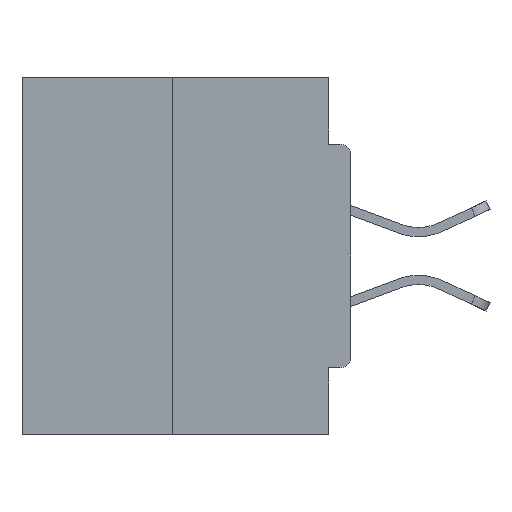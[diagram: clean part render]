
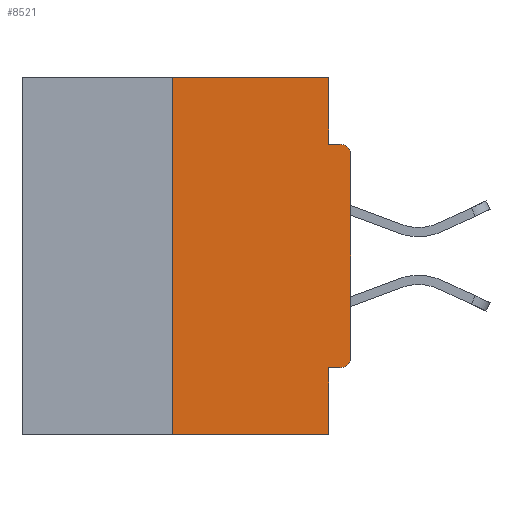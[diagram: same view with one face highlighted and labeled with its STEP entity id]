
A CAD part, left-side view. The second image highlights one B-rep face of the part: STEP entity #8521.
In plain terms, the highlighted planar face has unit normal (-1, 0, 0).
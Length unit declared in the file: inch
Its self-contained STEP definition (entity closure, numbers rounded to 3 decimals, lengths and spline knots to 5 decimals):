
#518 = LINE ( 'NONE', #33857, #13847 ) ;
#1133 = LINE ( 'NONE', #15920, #9068 ) ;
#1143 = CARTESIAN_POINT ( 'NONE',  ( 0., 0.031, -0.0935 ) ) ;
#1361 = VERTEX_POINT ( 'NONE', #1143 ) ;
#1629 = VECTOR ( 'NONE', #17990, 39.37008 ) ;
#2027 = EDGE_CURVE ( 'NONE', #19918, #19166, #31286, .T. ) ;
#2174 = CARTESIAN_POINT ( 'NONE',  ( 0., 0.015, -0.4065 ) ) ;
#2685 = DIRECTION ( 'NONE',  ( 0., 0., 1. ) ) ;
#2753 = DIRECTION ( 'NONE',  ( 0., 1., 0. ) ) ;
#2763 = FACE_OUTER_BOUND ( 'NONE', #19961, .T. ) ;
#3232 = ORIENTED_EDGE ( 'NONE', *, *, #8965, .T. ) ;
#3817 = ORIENTED_EDGE ( 'NONE', *, *, #30612, .F. ) ;
#4650 = CARTESIAN_POINT ( 'NONE',  ( 0., 0.25, -0.5 ) ) ;
#4652 = ORIENTED_EDGE ( 'NONE', *, *, #2027, .T. ) ;
#4657 = CARTESIAN_POINT ( 'NONE',  ( 0., 0.031, 0. ) ) ;
#4737 = DIRECTION ( 'NONE',  ( 0., -1., 0. ) ) ;
#4924 = EDGE_CURVE ( 'NONE', #19918, #27239, #34096, .T. ) ;
#4935 = CARTESIAN_POINT ( 'NONE',  ( 0., 0.031, -0.5 ) ) ;
#5098 = VERTEX_POINT ( 'NONE', #27482 ) ;
#7703 = EDGE_CURVE ( 'NONE', #1361, #5098, #30983, .T. ) ;
#7710 = CARTESIAN_POINT ( 'NONE',  ( 0., 0.46, 0. ) ) ;
#7733 = DIRECTION ( 'NONE',  ( 0., 0., -1. ) ) ;
#8521 = ADVANCED_FACE ( 'NONE', ( #2763 ), #30491, .F. ) ;
#8965 = EDGE_CURVE ( 'NONE', #17860, #16207, #21407, .T. ) ;
#9068 = VECTOR ( 'NONE', #2685, 39.37008 ) ;
#9953 = ORIENTED_EDGE ( 'NONE', *, *, #4924, .F. ) ;
#10108 = DIRECTION ( 'NONE',  ( 0., -1., 0. ) ) ;
#10559 = VECTOR ( 'NONE', #4737, 39.37008 ) ;
#11666 = CARTESIAN_POINT ( 'NONE',  ( 0., 0.031, -0.5 ) ) ;
#12344 = VECTOR ( 'NONE', #16666, 39.37008 ) ;
#12427 = EDGE_CURVE ( 'NONE', #32686, #5098, #20675, .T. ) ;
#13296 = DIRECTION ( 'NONE',  ( 0., 0., -1. ) ) ;
#13358 = CARTESIAN_POINT ( 'NONE',  ( 0., 0.031, -0.4065 ) ) ;
#13772 = ORIENTED_EDGE ( 'NONE', *, *, #26537, .T. ) ;
#13847 = VECTOR ( 'NONE', #10108, 39.37008 ) ;
#14230 = CARTESIAN_POINT ( 'NONE',  ( 0., 0., -0.0935 ) ) ;
#15646 = CARTESIAN_POINT ( 'NONE',  ( 0., 0., -0.4065 ) ) ;
#15920 = CARTESIAN_POINT ( 'NONE',  ( 0., 0., 0. ) ) ;
#16140 = ORIENTED_EDGE ( 'NONE', *, *, #32725, .F. ) ;
#16207 = VERTEX_POINT ( 'NONE', #24730 ) ;
#16448 = AXIS2_PLACEMENT_3D ( 'NONE', #7710, #28440, #20427 ) ;
#16666 = DIRECTION ( 'NONE',  ( 0., -1., 0. ) ) ;
#17650 = VECTOR ( 'NONE', #7733, 39.37008 ) ;
#17860 = VERTEX_POINT ( 'NONE', #2174 ) ;
#17990 = DIRECTION ( 'NONE',  ( 0., 0., -1. ) ) ;
#18476 = ORIENTED_EDGE ( 'NONE', *, *, #28109, .F. ) ;
#19166 = VERTEX_POINT ( 'NONE', #11666 ) ;
#19566 = ORIENTED_EDGE ( 'NONE', *, *, #12427, .T. ) ;
#19918 = VERTEX_POINT ( 'NONE', #4650 ) ;
#19961 = EDGE_LOOP ( 'NONE', ( #23922, #9953, #4652, #18476, #16140, #3232, #13772, #19566, #20881, #3817 ) ) ;
#20427 = DIRECTION ( 'NONE',  ( 0., 0., -1. ) ) ;
#20675 = CIRCLE ( 'NONE', #26813, 0.015 ) ;
#20879 = DIRECTION ( 'NONE',  ( 0., 0., 1. ) ) ;
#20881 = ORIENTED_EDGE ( 'NONE', *, *, #7703, .F. ) ;
#21407 = CIRCLE ( 'NONE', #23380, 0.015 ) ;
#22121 = CARTESIAN_POINT ( 'NONE',  ( 0., 0.031, 0. ) ) ;
#23380 = AXIS2_PLACEMENT_3D ( 'NONE', #31484, #23627, #13296 ) ;
#23459 = EDGE_CURVE ( 'NONE', #27239, #27442, #518, .T. ) ;
#23627 = DIRECTION ( 'NONE',  ( -1., 0., 0. ) ) ;
#23758 = DIRECTION ( 'NONE',  ( 0., 0., -1. ) ) ;
#23806 = CARTESIAN_POINT ( 'NONE',  ( 0., 0.25, 0. ) ) ;
#23922 = ORIENTED_EDGE ( 'NONE', *, *, #23459, .F. ) ;
#24006 = CARTESIAN_POINT ( 'NONE',  ( 0., 0.25, 0. ) ) ;
#24730 = CARTESIAN_POINT ( 'NONE',  ( 0., 0., -0.3915 ) ) ;
#26537 = EDGE_CURVE ( 'NONE', #16207, #32686, #1133, .T. ) ;
#26813 = AXIS2_PLACEMENT_3D ( 'NONE', #33908, #31357, #23758 ) ;
#27239 = VERTEX_POINT ( 'NONE', #24006 ) ;
#27442 = VERTEX_POINT ( 'NONE', #22121 ) ;
#27482 = CARTESIAN_POINT ( 'NONE',  ( 0., 0.015, -0.0935 ) ) ;
#28109 = EDGE_CURVE ( 'NONE', #28952, #19166, #30061, .T. ) ;
#28440 = DIRECTION ( 'NONE',  ( 1., 0., 0. ) ) ;
#28952 = VERTEX_POINT ( 'NONE', #13358 ) ;
#30061 = LINE ( 'NONE', #4935, #17650 ) ;
#30491 = PLANE ( 'NONE',  #16448 ) ;
#30612 = EDGE_CURVE ( 'NONE', #27442, #1361, #33192, .T. ) ;
#30929 = LINE ( 'NONE', #15646, #33836 ) ;
#30983 = LINE ( 'NONE', #14230, #12344 ) ;
#31030 = CARTESIAN_POINT ( 'NONE',  ( 0., 0.46, -0.5 ) ) ;
#31182 = VECTOR ( 'NONE', #20879, 39.37008 ) ;
#31286 = LINE ( 'NONE', #31030, #10559 ) ;
#31357 = DIRECTION ( 'NONE',  ( -1., 0., 0. ) ) ;
#31484 = CARTESIAN_POINT ( 'NONE',  ( 0., 0.015, -0.3915 ) ) ;
#31513 = CARTESIAN_POINT ( 'NONE',  ( 0., 0., -0.1085 ) ) ;
#32686 = VERTEX_POINT ( 'NONE', #31513 ) ;
#32725 = EDGE_CURVE ( 'NONE', #17860, #28952, #30929, .T. ) ;
#33192 = LINE ( 'NONE', #4657, #1629 ) ;
#33836 = VECTOR ( 'NONE', #2753, 39.37008 ) ;
#33857 = CARTESIAN_POINT ( 'NONE',  ( 0., 0.46, 0. ) ) ;
#33908 = CARTESIAN_POINT ( 'NONE',  ( 0., 0.015, -0.1085 ) ) ;
#34096 = LINE ( 'NONE', #23806, #31182 ) ;
